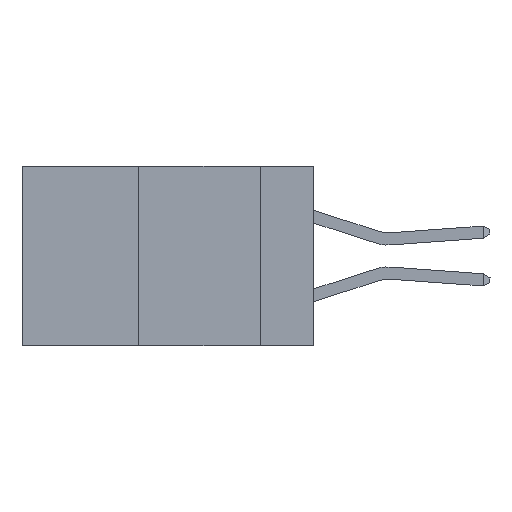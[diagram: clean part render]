
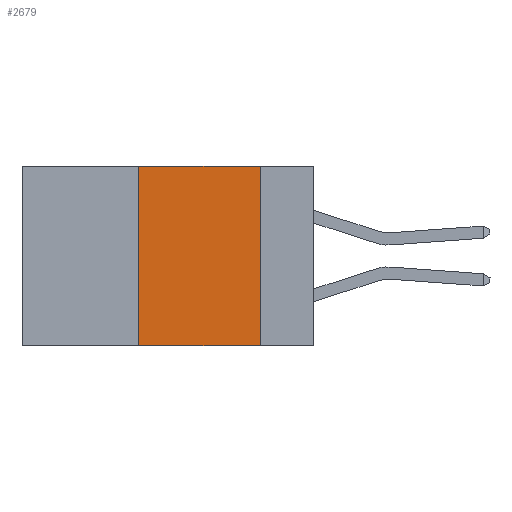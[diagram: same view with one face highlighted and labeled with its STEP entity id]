
A CAD part, left-side view. The second image highlights one B-rep face of the part: STEP entity #2679.
In plain terms, the highlighted planar face has unit normal (-1, 0, 0).
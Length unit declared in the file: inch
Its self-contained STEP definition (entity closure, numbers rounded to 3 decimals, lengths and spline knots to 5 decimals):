
#312 = CARTESIAN_POINT ( 'NONE',  ( 0., 0.36, 0. ) ) ;
#1068 = CARTESIAN_POINT ( 'NONE',  ( 0., 0.36, -0.37 ) ) ;
#2085 = AXIS2_PLACEMENT_3D ( 'NONE', #16961, #21046, #7526 ) ;
#2217 = LINE ( 'NONE', #16336, #8288 ) ;
#2679 = ADVANCED_FACE ( 'NONE', ( #11585 ), #17123, .F. ) ;
#2761 = VERTEX_POINT ( 'NONE', #19289 ) ;
#3025 = ORIENTED_EDGE ( 'NONE', *, *, #22831, .F. ) ;
#3229 = VECTOR ( 'NONE', #22072, 39.37008 ) ;
#3261 = ORIENTED_EDGE ( 'NONE', *, *, #24729, .F. ) ;
#4067 = ORIENTED_EDGE ( 'NONE', *, *, #12807, .F. ) ;
#4976 = LINE ( 'NONE', #21993, #16272 ) ;
#5981 = CARTESIAN_POINT ( 'NONE',  ( 0., 0.11, -0.37 ) ) ;
#7013 = VECTOR ( 'NONE', #24430, 39.37008 ) ;
#7526 = DIRECTION ( 'NONE',  ( 0., 0., -1. ) ) ;
#8288 = VECTOR ( 'NONE', #12646, 39.37008 ) ;
#11585 = FACE_OUTER_BOUND ( 'NONE', #20652, .T. ) ;
#12252 = DIRECTION ( 'NONE',  ( 0., 0., 1. ) ) ;
#12646 = DIRECTION ( 'NONE',  ( 0., -1., 0. ) ) ;
#12807 = EDGE_CURVE ( 'NONE', #16602, #2761, #20779, .T. ) ;
#13043 = VERTEX_POINT ( 'NONE', #5981 ) ;
#16272 = VECTOR ( 'NONE', #12252, 39.37008 ) ;
#16336 = CARTESIAN_POINT ( 'NONE',  ( 0., 0.6, -0.37 ) ) ;
#16602 = VERTEX_POINT ( 'NONE', #312 ) ;
#16961 = CARTESIAN_POINT ( 'NONE',  ( 0., 0.6, 0. ) ) ;
#17123 = PLANE ( 'NONE',  #2085 ) ;
#18520 = CARTESIAN_POINT ( 'NONE',  ( 0., 0.11, 0. ) ) ;
#18675 = CARTESIAN_POINT ( 'NONE',  ( 0., 0.6, 0. ) ) ;
#19289 = CARTESIAN_POINT ( 'NONE',  ( 0., 0.11, 0. ) ) ;
#20351 = LINE ( 'NONE', #18520, #3229 ) ;
#20652 = EDGE_LOOP ( 'NONE', ( #3025, #4067, #3261, #23040 ) ) ;
#20779 = LINE ( 'NONE', #18675, #7013 ) ;
#21046 = DIRECTION ( 'NONE',  ( 1., 0., 0. ) ) ;
#21993 = CARTESIAN_POINT ( 'NONE',  ( 0., 0.36, 0. ) ) ;
#22072 = DIRECTION ( 'NONE',  ( 0., 0., -1. ) ) ;
#22831 = EDGE_CURVE ( 'NONE', #2761, #13043, #20351, .T. ) ;
#23040 = ORIENTED_EDGE ( 'NONE', *, *, #24365, .T. ) ;
#24365 = EDGE_CURVE ( 'NONE', #24621, #13043, #2217, .T. ) ;
#24430 = DIRECTION ( 'NONE',  ( 0., -1., 0. ) ) ;
#24621 = VERTEX_POINT ( 'NONE', #1068 ) ;
#24729 = EDGE_CURVE ( 'NONE', #24621, #16602, #4976, .T. ) ;
